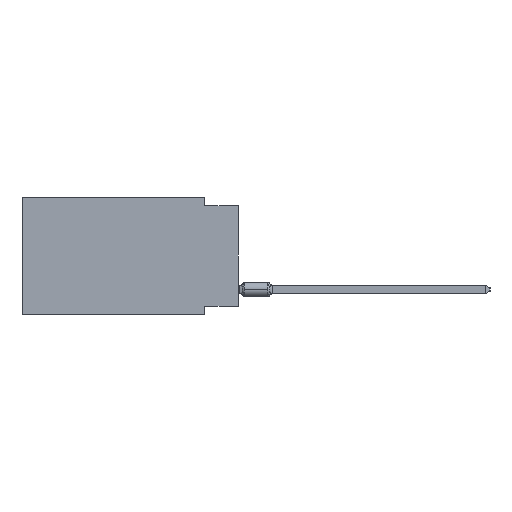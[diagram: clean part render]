
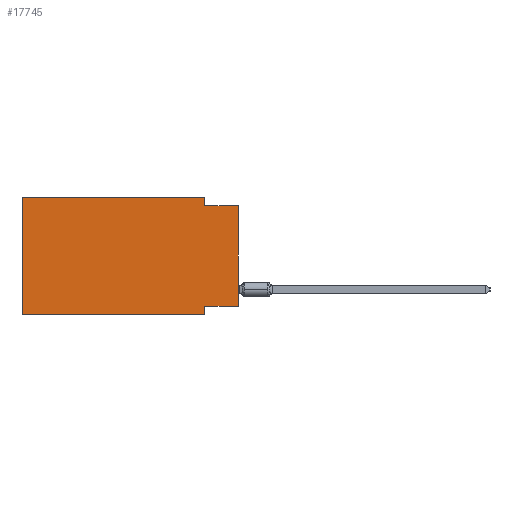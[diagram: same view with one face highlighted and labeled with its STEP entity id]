
A CAD part, left-side view. The second image highlights one B-rep face of the part: STEP entity #17745.
In plain terms, the highlighted planar face has unit normal (-1, 0, 0).
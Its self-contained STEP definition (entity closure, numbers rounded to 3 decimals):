
#728 = FACE_OUTER_BOUND ( 'NONE', #25072, .T. ) ;
#1324 = DIRECTION ( 'NONE',  ( 0., -1., 0. ) ) ;
#1427 = DIRECTION ( 'NONE',  ( 0., 0., -1. ) ) ;
#3956 = EDGE_CURVE ( 'NONE', #66161, #27454, #45013, .T. ) ;
#4701 = ORIENTED_EDGE ( 'NONE', *, *, #50117, .F. ) ;
#5615 = CARTESIAN_POINT ( 'NONE',  ( 0., 0., 0. ) ) ;
#9176 = DIRECTION ( 'NONE',  ( 0., -1., 0. ) ) ;
#10018 = LINE ( 'NONE', #41121, #42190 ) ;
#10835 = ORIENTED_EDGE ( 'NONE', *, *, #3956, .F. ) ;
#10922 = VECTOR ( 'NONE', #9176, 1000. ) ;
#11044 = LINE ( 'NONE', #36692, #12442 ) ;
#11187 = VECTOR ( 'NONE', #58250, 1000. ) ;
#11397 = CARTESIAN_POINT ( 'NONE',  ( 0., 2.54, -8.89 ) ) ;
#11833 = EDGE_CURVE ( 'NONE', #27874, #40955, #10018, .T. ) ;
#12442 = VECTOR ( 'NONE', #61989, 1000. ) ;
#13233 = EDGE_CURVE ( 'NONE', #40955, #51045, #67473, .T. ) ;
#13693 = CARTESIAN_POINT ( 'NONE',  ( 0., 0., -0.635 ) ) ;
#15726 = VERTEX_POINT ( 'NONE', #25031 ) ;
#17326 = VECTOR ( 'NONE', #57259, 1000. ) ;
#17745 = ADVANCED_FACE ( 'NONE', ( #728 ), #42814, .F. ) ;
#18788 = CARTESIAN_POINT ( 'NONE',  ( 0., 2.54, -8.255 ) ) ;
#18930 = DIRECTION ( 'NONE',  ( 0., 1., 0. ) ) ;
#19788 = CARTESIAN_POINT ( 'NONE',  ( 0., 16.383, -8.89 ) ) ;
#21034 = VECTOR ( 'NONE', #1324, 1000. ) ;
#23283 = LINE ( 'NONE', #13693, #53961 ) ;
#24940 = CARTESIAN_POINT ( 'NONE',  ( 0., 16.383, 0. ) ) ;
#25031 = CARTESIAN_POINT ( 'NONE',  ( 0., 0., -0.635 ) ) ;
#25072 = EDGE_LOOP ( 'NONE', ( #29057, #37268, #4701, #52315, #10835, #62400, #37613, #30361 ) ) ;
#25279 = AXIS2_PLACEMENT_3D ( 'NONE', #47593, #26390, #1427 ) ;
#26390 = DIRECTION ( 'NONE',  ( 1., 0., 0. ) ) ;
#26649 = CARTESIAN_POINT ( 'NONE',  ( 0., 16.383, -8.89 ) ) ;
#26930 = VERTEX_POINT ( 'NONE', #62613 ) ;
#27315 = CARTESIAN_POINT ( 'NONE',  ( 0., 16.383, 0. ) ) ;
#27454 = VERTEX_POINT ( 'NONE', #24940 ) ;
#27874 = VERTEX_POINT ( 'NONE', #56310 ) ;
#29057 = ORIENTED_EDGE ( 'NONE', *, *, #58104, .T. ) ;
#30361 = ORIENTED_EDGE ( 'NONE', *, *, #11833, .F. ) ;
#30519 = VECTOR ( 'NONE', #65844, 1000. ) ;
#34349 = CARTESIAN_POINT ( 'NONE',  ( 0., 2.54, -0.635 ) ) ;
#36692 = CARTESIAN_POINT ( 'NONE',  ( 0., 2.54, 0. ) ) ;
#36901 = LINE ( 'NONE', #27315, #21034 ) ;
#37268 = ORIENTED_EDGE ( 'NONE', *, *, #65862, .F. ) ;
#37613 = ORIENTED_EDGE ( 'NONE', *, *, #13233, .F. ) ;
#40955 = VERTEX_POINT ( 'NONE', #18788 ) ;
#41121 = CARTESIAN_POINT ( 'NONE',  ( 0., 0., -8.255 ) ) ;
#41532 = LINE ( 'NONE', #5615, #17326 ) ;
#42190 = VECTOR ( 'NONE', #18930, 1000. ) ;
#42814 = PLANE ( 'NONE',  #25279 ) ;
#43322 = VERTEX_POINT ( 'NONE', #34349 ) ;
#45013 = LINE ( 'NONE', #46013, #30519 ) ;
#46013 = CARTESIAN_POINT ( 'NONE',  ( 0., 16.383, 0. ) ) ;
#47593 = CARTESIAN_POINT ( 'NONE',  ( 0., 16.383, 0. ) ) ;
#50117 = EDGE_CURVE ( 'NONE', #26930, #43322, #11044, .T. ) ;
#50897 = LINE ( 'NONE', #19788, #10922 ) ;
#51045 = VERTEX_POINT ( 'NONE', #57949 ) ;
#52315 = ORIENTED_EDGE ( 'NONE', *, *, #54824, .F. ) ;
#53961 = VECTOR ( 'NONE', #55404, 1000. ) ;
#54824 = EDGE_CURVE ( 'NONE', #27454, #26930, #36901, .T. ) ;
#55404 = DIRECTION ( 'NONE',  ( 0., -1., 0. ) ) ;
#56310 = CARTESIAN_POINT ( 'NONE',  ( 0., 0., -8.255 ) ) ;
#57259 = DIRECTION ( 'NONE',  ( 0., 0., 1. ) ) ;
#57949 = CARTESIAN_POINT ( 'NONE',  ( 0., 2.54, -8.89 ) ) ;
#58104 = EDGE_CURVE ( 'NONE', #27874, #15726, #41532, .T. ) ;
#58250 = DIRECTION ( 'NONE',  ( 0., 0., -1. ) ) ;
#61081 = EDGE_CURVE ( 'NONE', #66161, #51045, #50897, .T. ) ;
#61989 = DIRECTION ( 'NONE',  ( 0., 0., -1. ) ) ;
#62400 = ORIENTED_EDGE ( 'NONE', *, *, #61081, .T. ) ;
#62613 = CARTESIAN_POINT ( 'NONE',  ( 0., 2.54, 0. ) ) ;
#65844 = DIRECTION ( 'NONE',  ( 0., 0., 1. ) ) ;
#65862 = EDGE_CURVE ( 'NONE', #43322, #15726, #23283, .T. ) ;
#66161 = VERTEX_POINT ( 'NONE', #26649 ) ;
#67473 = LINE ( 'NONE', #11397, #11187 ) ;
